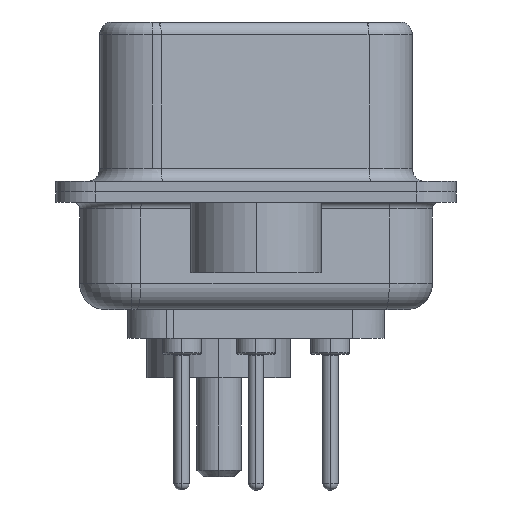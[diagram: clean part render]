
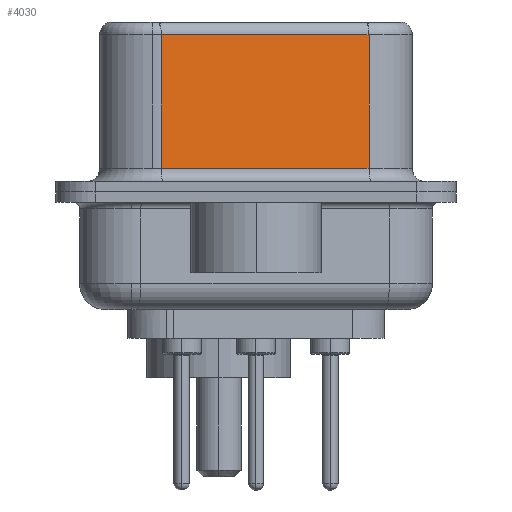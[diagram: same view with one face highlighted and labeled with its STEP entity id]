
A CAD part, left-side view. The second image highlights one B-rep face of the part: STEP entity #4030.
In plain terms, the highlighted planar face has unit normal (-0.985, -0.174, 0).
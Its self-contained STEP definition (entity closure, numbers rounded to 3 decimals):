
#726 = LINE ( 'NONE', #21322, #17748 ) ;
#1243 = CARTESIAN_POINT ( 'NONE',  ( 5.132, -4.322, 0.9 ) ) ;
#2439 = VECTOR ( 'NONE', #3478, 1000. ) ;
#2798 = DIRECTION ( 'NONE',  ( -0.174, 0.985, 0. ) ) ;
#3478 = DIRECTION ( 'NONE',  ( 0.174, -0.985, 0. ) ) ;
#4030 = ADVANCED_FACE ( 'NONE', ( #5884 ), #4566, .F. ) ;
#4214 = VECTOR ( 'NONE', #27987, 1000. ) ;
#4566 = PLANE ( 'NONE',  #23183 ) ;
#5877 = DIRECTION ( 'NONE',  ( 0., 0., -1. ) ) ;
#5884 = FACE_OUTER_BOUND ( 'NONE', #24856, .T. ) ;
#6860 = EDGE_CURVE ( 'NONE', #20490, #17693, #19906, .T. ) ;
#7433 = ORIENTED_EDGE ( 'NONE', *, *, #19579, .F. ) ;
#9061 = LINE ( 'NONE', #1243, #2439 ) ;
#9112 = VERTEX_POINT ( 'NONE', #23451 ) ;
#10125 = LINE ( 'NONE', #12595, #4214 ) ;
#12438 = EDGE_CURVE ( 'NONE', #17693, #9112, #726, .T. ) ;
#12595 = CARTESIAN_POINT ( 'NONE',  ( 5.132, -4.322, 6.52 ) ) ;
#13093 = EDGE_CURVE ( 'NONE', #9112, #22266, #9061, .T. ) ;
#13095 = ORIENTED_EDGE ( 'NONE', *, *, #12438, .T. ) ;
#17693 = VERTEX_POINT ( 'NONE', #19478 ) ;
#17741 = ORIENTED_EDGE ( 'NONE', *, *, #6860, .T. ) ;
#17748 = VECTOR ( 'NONE', #5877, 1000. ) ;
#18044 = ORIENTED_EDGE ( 'NONE', *, *, #13093, .T. ) ;
#19478 = CARTESIAN_POINT ( 'NONE',  ( 3.73, 3.628, 6.02 ) ) ;
#19579 = EDGE_CURVE ( 'NONE', #20490, #22266, #10125, .T. ) ;
#19906 = LINE ( 'NONE', #24427, #25011 ) ;
#20490 = VERTEX_POINT ( 'NONE', #24475 ) ;
#21322 = CARTESIAN_POINT ( 'NONE',  ( 3.73, 3.628, 6.52 ) ) ;
#22266 = VERTEX_POINT ( 'NONE', #24787 ) ;
#23183 = AXIS2_PLACEMENT_3D ( 'NONE', #28001, #28499, #2798 ) ;
#23451 = CARTESIAN_POINT ( 'NONE',  ( 3.73, 3.628, 0.9 ) ) ;
#24427 = CARTESIAN_POINT ( 'NONE',  ( 5.132, -4.322, 6.02 ) ) ;
#24475 = CARTESIAN_POINT ( 'NONE',  ( 5.132, -4.322, 6.02 ) ) ;
#24787 = CARTESIAN_POINT ( 'NONE',  ( 5.132, -4.322, 0.9 ) ) ;
#24856 = EDGE_LOOP ( 'NONE', ( #7433, #17741, #13095, #18044 ) ) ;
#25011 = VECTOR ( 'NONE', #28253, 1000. ) ;
#27987 = DIRECTION ( 'NONE',  ( 0., 0., -1. ) ) ;
#28001 = CARTESIAN_POINT ( 'NONE',  ( 5.132, -4.322, 6.52 ) ) ;
#28253 = DIRECTION ( 'NONE',  ( -0.174, 0.985, 0. ) ) ;
#28499 = DIRECTION ( 'NONE',  ( 0.985, 0.174, 0. ) ) ;
